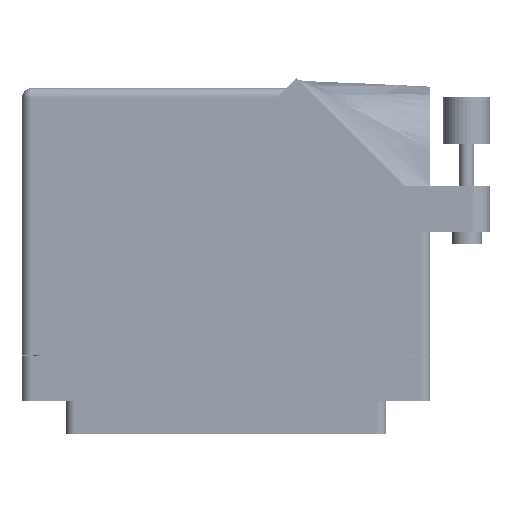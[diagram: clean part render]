
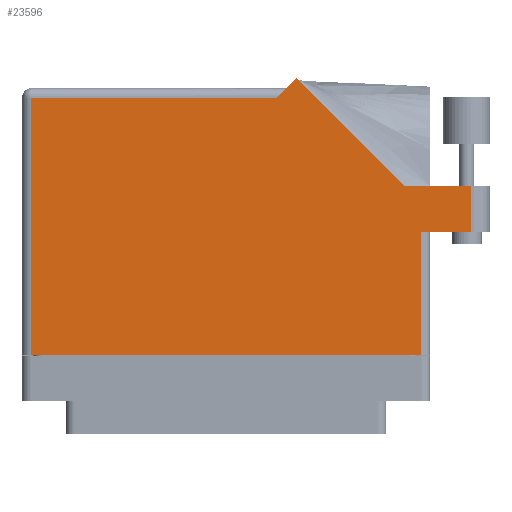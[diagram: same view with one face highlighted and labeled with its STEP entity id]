
A CAD part, front view. The second image highlights one B-rep face of the part: STEP entity #23596.
In plain terms, the highlighted face is planar.
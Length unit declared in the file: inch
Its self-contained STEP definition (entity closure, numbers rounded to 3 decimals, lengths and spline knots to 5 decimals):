
#3648 = DIRECTION ( 'NONE',  ( -1., 0., 0. ) ) ;
#4619 = LINE ( 'NONE', #10013, #52702 ) ;
#4774 = EDGE_CURVE ( 'NONE', #24964, #58588, #67378, .T. ) ;
#5591 = CARTESIAN_POINT ( 'NONE',  ( 1.297, -0.1, 0.617 ) ) ;
#7506 = CARTESIAN_POINT ( 'NONE',  ( 1.297, 0.715, 0.617 ) ) ;
#7937 = LINE ( 'NONE', #34787, #29303 ) ;
#8065 = VECTOR ( 'NONE', #50129, 39.37008 ) ;
#8276 = DIRECTION ( 'NONE',  ( -1., 0., 0. ) ) ;
#10013 = CARTESIAN_POINT ( 'NONE',  ( -1.359, 1.613, 0.617 ) ) ;
#10355 = EDGE_CURVE ( 'NONE', #54017, #38665, #24966, .T. ) ;
#10389 = CARTESIAN_POINT ( 'NONE',  ( -1.297, -0.1, 0.617 ) ) ;
#12749 = EDGE_CURVE ( 'NONE', #25396, #54017, #42358, .T. ) ;
#13710 = VECTOR ( 'NONE', #46844, 39.37008 ) ;
#15516 = ORIENTED_EDGE ( 'NONE', *, *, #34968, .T. ) ;
#17779 = VECTOR ( 'NONE', #41779, 39.37008 ) ;
#19316 = CARTESIAN_POINT ( 'NONE',  ( -1.359, -0.1, 0.617 ) ) ;
#19848 = VERTEX_POINT ( 'NONE', #44802 ) ;
#21123 = CARTESIAN_POINT ( 'NONE',  ( 1.19342, 1.022, 0.617 ) ) ;
#23596 = ADVANCED_FACE ( 'NONE', ( #38110 ), #36663, .F. ) ;
#23625 = DIRECTION ( 'NONE',  ( -0.707, -0.707, 0. ) ) ;
#24964 = VERTEX_POINT ( 'NONE', #65455 ) ;
#24966 = LINE ( 'NONE', #25133, #17779 ) ;
#25133 = CARTESIAN_POINT ( 'NONE',  ( 1.297, 0.715, 0.617 ) ) ;
#25396 = VERTEX_POINT ( 'NONE', #10389 ) ;
#26728 = EDGE_CURVE ( 'NONE', #71336, #19848, #43969, .T. ) ;
#27227 = VECTOR ( 'NONE', #70914, 39.37008 ) ;
#27726 = VECTOR ( 'NONE', #44641, 39.37008 ) ;
#29303 = VECTOR ( 'NONE', #23625, 39.37008 ) ;
#31068 = EDGE_CURVE ( 'NONE', #19848, #24964, #65622, .T. ) ;
#32073 = AXIS2_PLACEMENT_3D ( 'NONE', #42393, #53077, #8276 ) ;
#34233 = EDGE_CURVE ( 'NONE', #43538, #25396, #64263, .T. ) ;
#34662 = CARTESIAN_POINT ( 'NONE',  ( 0.337, 1.613, 0.617 ) ) ;
#34787 = CARTESIAN_POINT ( 'NONE',  ( 0.399, 1.675, 0.617 ) ) ;
#34968 = EDGE_CURVE ( 'NONE', #38665, #71336, #60550, .T. ) ;
#36663 = PLANE ( 'NONE',  #32073 ) ;
#38110 = FACE_OUTER_BOUND ( 'NONE', #49514, .T. ) ;
#38665 = VERTEX_POINT ( 'NONE', #7506 ) ;
#38704 = CARTESIAN_POINT ( 'NONE',  ( 1.359, 0.715, 0.617 ) ) ;
#39014 = ORIENTED_EDGE ( 'NONE', *, *, #12749, .T. ) ;
#41779 = DIRECTION ( 'NONE',  ( 0., 1., 0. ) ) ;
#42358 = LINE ( 'NONE', #19316, #27227 ) ;
#42393 = CARTESIAN_POINT ( 'NONE',  ( -1.359, 1.675, 0.617 ) ) ;
#42866 = ORIENTED_EDGE ( 'NONE', *, *, #26728, .T. ) ;
#42906 = ORIENTED_EDGE ( 'NONE', *, *, #34233, .T. ) ;
#42909 = CARTESIAN_POINT ( 'NONE',  ( -1.297, -0.1, 0.617 ) ) ;
#43538 = VERTEX_POINT ( 'NONE', #47669 ) ;
#43786 = ORIENTED_EDGE ( 'NONE', *, *, #31068, .T. ) ;
#43969 = LINE ( 'NONE', #59270, #13710 ) ;
#44641 = DIRECTION ( 'NONE',  ( 0., -1., 0. ) ) ;
#44802 = CARTESIAN_POINT ( 'NONE',  ( 1.634, 1.022, 0.617 ) ) ;
#46434 = EDGE_CURVE ( 'NONE', #70568, #43538, #4619, .T. ) ;
#46844 = DIRECTION ( 'NONE',  ( 0., 1., 0. ) ) ;
#47669 = CARTESIAN_POINT ( 'NONE',  ( -1.297, 1.613, 0.617 ) ) ;
#49514 = EDGE_LOOP ( 'NONE', ( #15516, #42866, #43786, #72322, #65557, #69904, #42906, #39014, #54527 ) ) ;
#49713 = EDGE_CURVE ( 'NONE', #58588, #70568, #7937, .T. ) ;
#49951 = DIRECTION ( 'NONE',  ( -0.707, 0.707, 0. ) ) ;
#50129 = DIRECTION ( 'NONE',  ( 1., 0., 0. ) ) ;
#52702 = VECTOR ( 'NONE', #54844, 39.37008 ) ;
#53077 = DIRECTION ( 'NONE',  ( 0., 0., -1. ) ) ;
#54017 = VERTEX_POINT ( 'NONE', #5591 ) ;
#54527 = ORIENTED_EDGE ( 'NONE', *, *, #10355, .T. ) ;
#54844 = DIRECTION ( 'NONE',  ( -1., 0., 0. ) ) ;
#58588 = VERTEX_POINT ( 'NONE', #72719 ) ;
#59262 = VECTOR ( 'NONE', #49951, 39.37008 ) ;
#59270 = CARTESIAN_POINT ( 'NONE',  ( 1.634, 1.022, 0.617 ) ) ;
#60550 = LINE ( 'NONE', #38704, #8065 ) ;
#60688 = CARTESIAN_POINT ( 'NONE',  ( 1.634, 0.715, 0.617 ) ) ;
#64263 = LINE ( 'NONE', #42909, #27726 ) ;
#65455 = CARTESIAN_POINT ( 'NONE',  ( 1.19342, 1.022, 0.617 ) ) ;
#65557 = ORIENTED_EDGE ( 'NONE', *, *, #49713, .T. ) ;
#65622 = LINE ( 'NONE', #72471, #71859 ) ;
#67378 = LINE ( 'NONE', #21123, #59262 ) ;
#69904 = ORIENTED_EDGE ( 'NONE', *, *, #46434, .T. ) ;
#70568 = VERTEX_POINT ( 'NONE', #34662 ) ;
#70914 = DIRECTION ( 'NONE',  ( 1., 0., 0. ) ) ;
#71336 = VERTEX_POINT ( 'NONE', #60688 ) ;
#71859 = VECTOR ( 'NONE', #3648, 39.37008 ) ;
#72322 = ORIENTED_EDGE ( 'NONE', *, *, #4774, .T. ) ;
#72471 = CARTESIAN_POINT ( 'NONE',  ( 1.759, 1.022, 0.617 ) ) ;
#72719 = CARTESIAN_POINT ( 'NONE',  ( 0.46971, 1.74571, 0.617 ) ) ;
